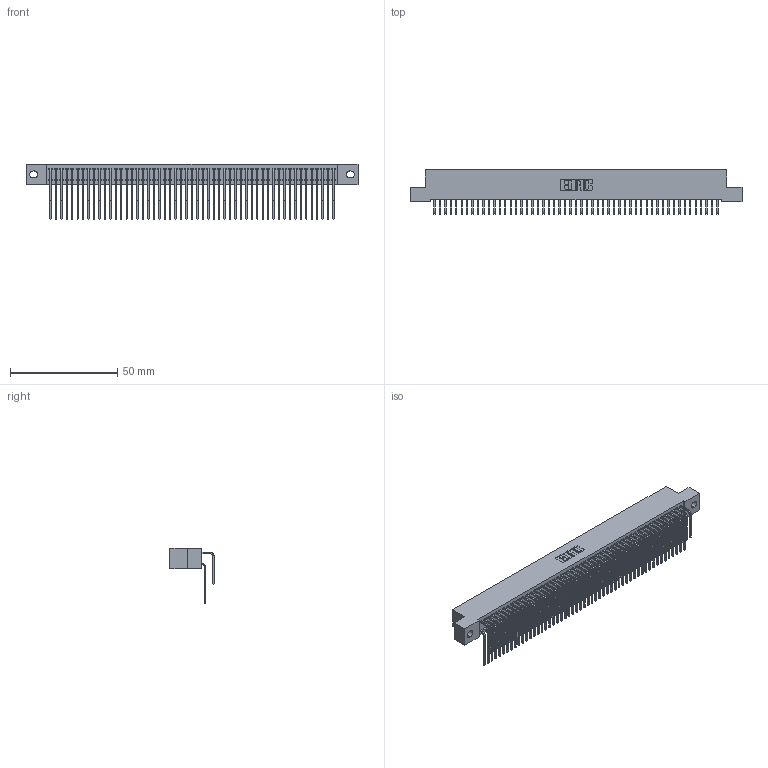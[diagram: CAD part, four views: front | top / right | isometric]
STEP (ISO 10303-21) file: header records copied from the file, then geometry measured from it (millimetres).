
FILE_DESCRIPTION (( 'STEP AP203' ), '1' );
FILE_NAME ('392-106-559-202.STEP', '2019-10-09T22:50:00', ( '' ), ( '' ), 'SwSTEP 2.0', 'SolidWorks 2016', '' );
FILE_SCHEMA (( 'CONFIG_CONTROL_DESIGN' ));
Length unit declared in the file: inch
Products named in the file (4): 342 Part_.128 Slot; 345-292-001_558 559 Tail - 1; 345-292-001_559 Tail - 2; 392-106-559-202
Assembly tree (107 placements, depth 2):
  392-106-559-202
    342 Part_.128 Slot
    345-292-001_558 559 Tail - 1  x53
    345-292-001_559 Tail - 2  x53
Bounding box: 154.94 x 20.64 x 25.78 mm (x, y, z)
Volume: 14532.7 mm3; surface area: 26452.3 mm2
Topology: 107 solids, 107 shells, 5838 faces, 17377 edges, 11442 vertices
Faces by surface type: plane 4098, cylinder 1740
Entity records: 34461 total; most frequent: CARTESIAN_POINT 5749, ORIENTED_EDGE 5634, DIRECTION 4873, EDGE_CURVE 2817, LINE 2649, VECTOR 2649, VERTEX_POINT 1874, AXIS2_PLACEMENT_3D 1112
